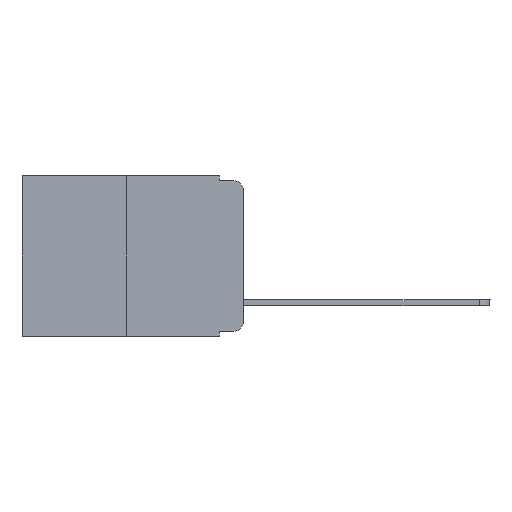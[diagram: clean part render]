
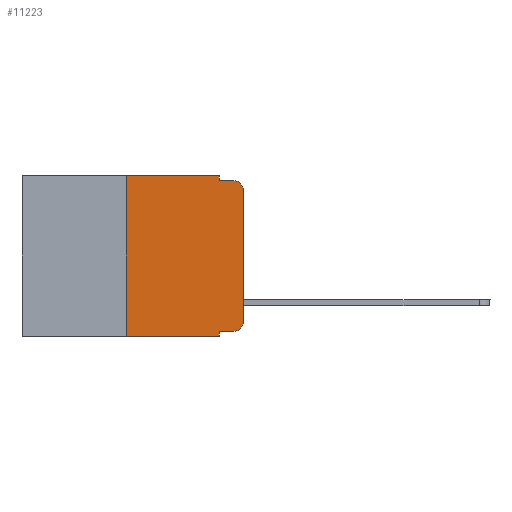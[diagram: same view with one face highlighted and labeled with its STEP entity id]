
A CAD part, left-side view. The second image highlights one B-rep face of the part: STEP entity #11223.
In plain terms, the highlighted planar face has unit normal (-1, 0, 0).
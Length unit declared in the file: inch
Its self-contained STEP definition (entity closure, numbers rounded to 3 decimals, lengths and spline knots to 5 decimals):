
#151 = CARTESIAN_POINT ( 'NONE',  ( 0., 0.25, 0. ) ) ;
#301 = CARTESIAN_POINT ( 'NONE',  ( 0., 0.02, -0.333 ) ) ;
#491 = ORIENTED_EDGE ( 'NONE', *, *, #10253, .F. ) ;
#558 = DIRECTION ( 'NONE',  ( 0., 0., -1. ) ) ;
#863 = ORIENTED_EDGE ( 'NONE', *, *, #10792, .T. ) ;
#1114 = VECTOR ( 'NONE', #6344, 39.37008 ) ;
#1785 = CARTESIAN_POINT ( 'NONE',  ( 0., 0., 0. ) ) ;
#1794 = VERTEX_POINT ( 'NONE', #2409 ) ;
#2093 = DIRECTION ( 'NONE',  ( 0., 0., -1. ) ) ;
#2162 = DIRECTION ( 'NONE',  ( -1., 0., 0. ) ) ;
#2328 = CARTESIAN_POINT ( 'NONE',  ( 0., 0., -0.03 ) ) ;
#2409 = CARTESIAN_POINT ( 'NONE',  ( 0., 0.02, -0.01 ) ) ;
#2685 = EDGE_CURVE ( 'NONE', #13656, #13278, #14684, .T. ) ;
#2823 = CARTESIAN_POINT ( 'NONE',  ( 0., 0.051, -0.343 ) ) ;
#3602 = EDGE_CURVE ( 'NONE', #17274, #9200, #9913, .T. ) ;
#3795 = LINE ( 'NONE', #10274, #1114 ) ;
#3908 = CARTESIAN_POINT ( 'NONE',  ( 0., 0.473, -0.343 ) ) ;
#4444 = DIRECTION ( 'NONE',  ( 1., 0., 0. ) ) ;
#4786 = CARTESIAN_POINT ( 'NONE',  ( 0., 0.02, -0.03 ) ) ;
#4992 = ORIENTED_EDGE ( 'NONE', *, *, #13116, .T. ) ;
#5105 = LINE ( 'NONE', #3908, #10793 ) ;
#5871 = EDGE_CURVE ( 'NONE', #13219, #13656, #14014, .T. ) ;
#5920 = VECTOR ( 'NONE', #7550, 39.37008 ) ;
#6207 = ORIENTED_EDGE ( 'NONE', *, *, #8148, .F. ) ;
#6280 = CARTESIAN_POINT ( 'NONE',  ( 0., 0.02, -0.313 ) ) ;
#6344 = DIRECTION ( 'NONE',  ( 0., 0., -1. ) ) ;
#6403 = EDGE_CURVE ( 'NONE', #7371, #1794, #8302, .T. ) ;
#6631 = VECTOR ( 'NONE', #9591, 39.37008 ) ;
#6736 = CIRCLE ( 'NONE', #6974, 0.02 ) ;
#6974 = AXIS2_PLACEMENT_3D ( 'NONE', #4786, #8547, #558 ) ;
#7142 = CARTESIAN_POINT ( 'NONE',  ( 0., 0.473, 0. ) ) ;
#7350 = CARTESIAN_POINT ( 'NONE',  ( 0., 0., -0.313 ) ) ;
#7371 = VERTEX_POINT ( 'NONE', #13140 ) ;
#7550 = DIRECTION ( 'NONE',  ( 0., -1., 0. ) ) ;
#7825 = ORIENTED_EDGE ( 'NONE', *, *, #6403, .F. ) ;
#8148 = EDGE_CURVE ( 'NONE', #9200, #7371, #16869, .T. ) ;
#8302 = LINE ( 'NONE', #16337, #6631 ) ;
#8372 = VERTEX_POINT ( 'NONE', #2823 ) ;
#8547 = DIRECTION ( 'NONE',  ( -1., 0., 0. ) ) ;
#8596 = ORIENTED_EDGE ( 'NONE', *, *, #2685, .T. ) ;
#9200 = VERTEX_POINT ( 'NONE', #11937 ) ;
#9211 = VERTEX_POINT ( 'NONE', #10660 ) ;
#9268 = EDGE_CURVE ( 'NONE', #9211, #8372, #5105, .T. ) ;
#9591 = DIRECTION ( 'NONE',  ( 0., -1., 0. ) ) ;
#9604 = VECTOR ( 'NONE', #16717, 39.37008 ) ;
#9771 = DIRECTION ( 'NONE',  ( 0., 0., 1. ) ) ;
#9782 = AXIS2_PLACEMENT_3D ( 'NONE', #7142, #4444, #13856 ) ;
#9913 = LINE ( 'NONE', #15464, #5920 ) ;
#10253 = EDGE_CURVE ( 'NONE', #13219, #8372, #3795, .T. ) ;
#10274 = CARTESIAN_POINT ( 'NONE',  ( 0., 0.051, 0. ) ) ;
#10427 = VECTOR ( 'NONE', #13967, 39.37008 ) ;
#10660 = CARTESIAN_POINT ( 'NONE',  ( 0., 0.25, -0.343 ) ) ;
#10792 = EDGE_CURVE ( 'NONE', #13497, #1794, #6736, .T. ) ;
#10793 = VECTOR ( 'NONE', #14786, 39.37008 ) ;
#11030 = VECTOR ( 'NONE', #13401, 39.37008 ) ;
#11132 = CARTESIAN_POINT ( 'NONE',  ( 0., 0.051, -0.333 ) ) ;
#11223 = ADVANCED_FACE ( 'NONE', ( #17178 ), #15200, .F. ) ;
#11937 = CARTESIAN_POINT ( 'NONE',  ( 0., 0.051, 0. ) ) ;
#12095 = ORIENTED_EDGE ( 'NONE', *, *, #3602, .F. ) ;
#12591 = CARTESIAN_POINT ( 'NONE',  ( 0., 0.25, 0. ) ) ;
#12727 = EDGE_LOOP ( 'NONE', ( #4992, #863, #7825, #6207, #12095, #16403, #15940, #491, #13964, #8596 ) ) ;
#13116 = EDGE_CURVE ( 'NONE', #13278, #13497, #14850, .T. ) ;
#13140 = CARTESIAN_POINT ( 'NONE',  ( 0., 0.051, -0.01 ) ) ;
#13219 = VERTEX_POINT ( 'NONE', #15232 ) ;
#13278 = VERTEX_POINT ( 'NONE', #7350 ) ;
#13285 = EDGE_CURVE ( 'NONE', #9211, #17274, #15688, .T. ) ;
#13401 = DIRECTION ( 'NONE',  ( 0., 0., -1. ) ) ;
#13497 = VERTEX_POINT ( 'NONE', #2328 ) ;
#13656 = VERTEX_POINT ( 'NONE', #301 ) ;
#13856 = DIRECTION ( 'NONE',  ( 0., 0., -1. ) ) ;
#13892 = AXIS2_PLACEMENT_3D ( 'NONE', #6280, #2162, #2093 ) ;
#13964 = ORIENTED_EDGE ( 'NONE', *, *, #5871, .T. ) ;
#13967 = DIRECTION ( 'NONE',  ( 0., -1., 0. ) ) ;
#14014 = LINE ( 'NONE', #11132, #10427 ) ;
#14440 = VECTOR ( 'NONE', #9771, 39.37008 ) ;
#14461 = CARTESIAN_POINT ( 'NONE',  ( 0., 0.051, 0. ) ) ;
#14684 = CIRCLE ( 'NONE', #13892, 0.02 ) ;
#14786 = DIRECTION ( 'NONE',  ( 0., -1., 0. ) ) ;
#14850 = LINE ( 'NONE', #1785, #14440 ) ;
#15200 = PLANE ( 'NONE',  #9782 ) ;
#15232 = CARTESIAN_POINT ( 'NONE',  ( 0., 0.051, -0.333 ) ) ;
#15464 = CARTESIAN_POINT ( 'NONE',  ( 0., 0.473, 0. ) ) ;
#15688 = LINE ( 'NONE', #12591, #9604 ) ;
#15940 = ORIENTED_EDGE ( 'NONE', *, *, #9268, .T. ) ;
#16337 = CARTESIAN_POINT ( 'NONE',  ( 0., 0.051, -0.01 ) ) ;
#16403 = ORIENTED_EDGE ( 'NONE', *, *, #13285, .F. ) ;
#16717 = DIRECTION ( 'NONE',  ( 0., 0., 1. ) ) ;
#16869 = LINE ( 'NONE', #14461, #11030 ) ;
#17178 = FACE_OUTER_BOUND ( 'NONE', #12727, .T. ) ;
#17274 = VERTEX_POINT ( 'NONE', #151 ) ;
